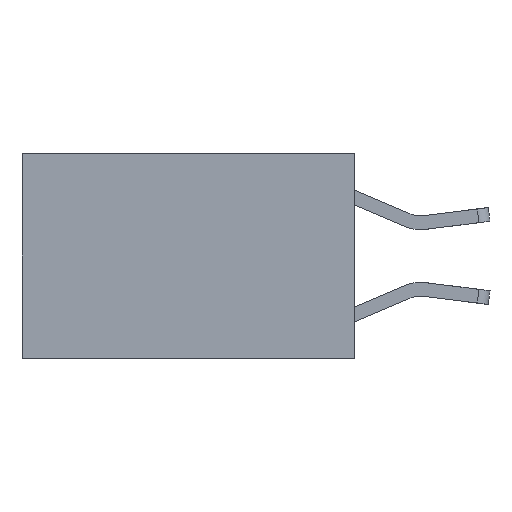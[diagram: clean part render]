
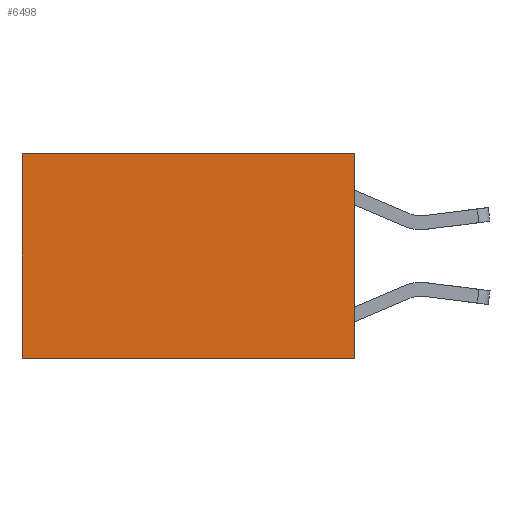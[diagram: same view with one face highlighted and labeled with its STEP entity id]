
A CAD part, left-side view. The second image highlights one B-rep face of the part: STEP entity #6498.
In plain terms, the highlighted planar face has unit normal (-1, 0, 0).
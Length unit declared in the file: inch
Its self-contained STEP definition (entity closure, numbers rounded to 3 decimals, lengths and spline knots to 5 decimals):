
#215 = DIRECTION ( 'NONE',  ( 0., 1., 0. ) ) ;
#225 = ORIENTED_EDGE ( 'NONE', *, *, #862, .T. ) ;
#296 = CARTESIAN_POINT ( 'NONE',  ( 0.2625, 0., -0.37 ) ) ;
#340 = PLANE ( 'NONE',  #3428 ) ;
#415 = LINE ( 'NONE', #7351, #7761 ) ;
#449 = EDGE_CURVE ( 'NONE', #1912, #4957, #6584, .T. ) ;
#862 = EDGE_CURVE ( 'NONE', #1633, #1910, #3689, .T. ) ;
#962 = CARTESIAN_POINT ( 'NONE',  ( 0.2625, 0., 0. ) ) ;
#1633 = VERTEX_POINT ( 'NONE', #1861 ) ;
#1843 = ORIENTED_EDGE ( 'NONE', *, *, #4228, .T. ) ;
#1861 = CARTESIAN_POINT ( 'NONE',  ( 0.2625, 0., 0. ) ) ;
#1910 = VERTEX_POINT ( 'NONE', #2728 ) ;
#1912 = VERTEX_POINT ( 'NONE', #296 ) ;
#2728 = CARTESIAN_POINT ( 'NONE',  ( 0.2625, 0.6, 0. ) ) ;
#2900 = CARTESIAN_POINT ( 'NONE',  ( 0.2625, 0., -0.37 ) ) ;
#3427 = CARTESIAN_POINT ( 'NONE',  ( 0.2625, 0., 0. ) ) ;
#3428 = AXIS2_PLACEMENT_3D ( 'NONE', #6387, #8378, #4391 ) ;
#3463 = DIRECTION ( 'NONE',  ( 0., 0., -1. ) ) ;
#3689 = LINE ( 'NONE', #962, #5239 ) ;
#4228 = EDGE_CURVE ( 'NONE', #1910, #4957, #415, .T. ) ;
#4391 = DIRECTION ( 'NONE',  ( 0., 0., -1. ) ) ;
#4468 = VECTOR ( 'NONE', #3463, 39.37008 ) ;
#4957 = VERTEX_POINT ( 'NONE', #7700 ) ;
#5239 = VECTOR ( 'NONE', #6115, 39.37008 ) ;
#5392 = ORIENTED_EDGE ( 'NONE', *, *, #6117, .F. ) ;
#5569 = ORIENTED_EDGE ( 'NONE', *, *, #449, .F. ) ;
#6115 = DIRECTION ( 'NONE',  ( 0., 1., 0. ) ) ;
#6117 = EDGE_CURVE ( 'NONE', #1633, #1912, #8042, .T. ) ;
#6169 = VECTOR ( 'NONE', #215, 39.37008 ) ;
#6387 = CARTESIAN_POINT ( 'NONE',  ( 0.2625, 0., 0. ) ) ;
#6498 = ADVANCED_FACE ( 'NONE', ( #7077 ), #340, .F. ) ;
#6584 = LINE ( 'NONE', #2900, #6169 ) ;
#7024 = EDGE_LOOP ( 'NONE', ( #1843, #5569, #5392, #225 ) ) ;
#7077 = FACE_OUTER_BOUND ( 'NONE', #7024, .T. ) ;
#7351 = CARTESIAN_POINT ( 'NONE',  ( 0.2625, 0.6, 0. ) ) ;
#7700 = CARTESIAN_POINT ( 'NONE',  ( 0.2625, 0.6, -0.37 ) ) ;
#7761 = VECTOR ( 'NONE', #8512, 39.37008 ) ;
#8042 = LINE ( 'NONE', #3427, #4468 ) ;
#8378 = DIRECTION ( 'NONE',  ( 1., 0., 0. ) ) ;
#8512 = DIRECTION ( 'NONE',  ( 0., 0., -1. ) ) ;
